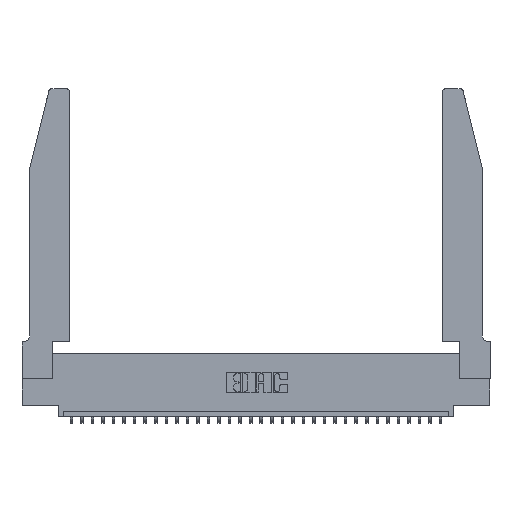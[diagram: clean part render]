
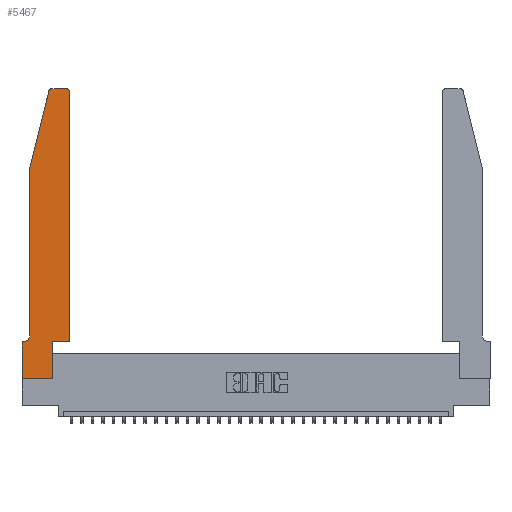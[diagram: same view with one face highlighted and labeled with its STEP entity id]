
A CAD part, top view. The second image highlights one B-rep face of the part: STEP entity #5467.
In plain terms, the highlighted planar face has unit normal (0, 0, 1).
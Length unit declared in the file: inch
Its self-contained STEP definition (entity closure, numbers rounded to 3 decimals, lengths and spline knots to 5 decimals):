
#91 = CARTESIAN_POINT ( 'NONE',  ( 0., 0., 0.37 ) ) ;
#189 = DIRECTION ( 'NONE',  ( 1., 0., 0. ) ) ;
#354 = VERTEX_POINT ( 'NONE', #4763 ) ;
#559 = AXIS2_PLACEMENT_3D ( 'NONE', #20808, #7820, #15425 ) ;
#624 = EDGE_CURVE ( 'NONE', #32583, #28221, #8043, .T. ) ;
#1134 = CARTESIAN_POINT ( 'NONE',  ( 0.2865, 0., 0.37 ) ) ;
#1502 = CARTESIAN_POINT ( 'NONE',  ( 0.284, 2.72, 0.37 ) ) ;
#1786 = AXIS2_PLACEMENT_3D ( 'NONE', #6317, #21742, #11799 ) ;
#2083 = CARTESIAN_POINT ( 'NONE',  ( 0.4505, 0.35, 0.37 ) ) ;
#2113 = EDGE_CURVE ( 'NONE', #14471, #32750, #32723, .T. ) ;
#2166 = DIRECTION ( 'NONE',  ( -1., 0., 0. ) ) ;
#2376 = CARTESIAN_POINT ( 'NONE',  ( 0.0755, 0.35, 0.37 ) ) ;
#2480 = CIRCLE ( 'NONE', #9374, 0.07 ) ;
#3508 = EDGE_CURVE ( 'NONE', #17828, #15352, #21882, .T. ) ;
#4002 = CIRCLE ( 'NONE', #26710, 0.03 ) ;
#4449 = CARTESIAN_POINT ( 'NONE',  ( 0.2865, 0.35, 0.37 ) ) ;
#4587 = VECTOR ( 'NONE', #30036, 39.37008 ) ;
#4680 = DIRECTION ( 'NONE',  ( 0., 1., 0. ) ) ;
#4698 = EDGE_CURVE ( 'NONE', #22124, #354, #21818, .T. ) ;
#4763 = CARTESIAN_POINT ( 'NONE',  ( 0.2865, 0.35, 0.37 ) ) ;
#5367 = CARTESIAN_POINT ( 'NONE',  ( 0.284, 2.75, 0.37 ) ) ;
#5467 = ADVANCED_FACE ( 'NONE', ( #28882 ), #31839, .T. ) ;
#5757 = ORIENTED_EDGE ( 'NONE', *, *, #4698, .T. ) ;
#6317 = CARTESIAN_POINT ( 'NONE',  ( 0., 0.35, 0.37 ) ) ;
#7056 = CARTESIAN_POINT ( 'NONE',  ( 0.4505, 0.35, 0.37 ) ) ;
#7820 = DIRECTION ( 'NONE',  ( 0., 0., 1. ) ) ;
#8043 = LINE ( 'NONE', #14419, #28275 ) ;
#8946 = VECTOR ( 'NONE', #189, 39.37008 ) ;
#9374 = AXIS2_PLACEMENT_3D ( 'NONE', #27541, #12500, #2166 ) ;
#9375 = LINE ( 'NONE', #2083, #4587 ) ;
#9387 = EDGE_CURVE ( 'NONE', #354, #25206, #22438, .T. ) ;
#9686 = CARTESIAN_POINT ( 'NONE',  ( 0., 0., 0.37 ) ) ;
#9742 = VECTOR ( 'NONE', #18309, 39.37008 ) ;
#9914 = DIRECTION ( 'NONE',  ( -1., 0., 0. ) ) ;
#9965 = DIRECTION ( 'NONE',  ( 0., 0., 1. ) ) ;
#10332 = ORIENTED_EDGE ( 'NONE', *, *, #15098, .T. ) ;
#10562 = DIRECTION ( 'NONE',  ( -0.239, -0.971, 0. ) ) ;
#10989 = ORIENTED_EDGE ( 'NONE', *, *, #12234, .T. ) ;
#11799 = DIRECTION ( 'NONE',  ( 1., 0., 0. ) ) ;
#12012 = DIRECTION ( 'NONE',  ( -1., 0., 0. ) ) ;
#12234 = EDGE_CURVE ( 'NONE', #12552, #17828, #25350, .T. ) ;
#12296 = DIRECTION ( 'NONE',  ( 1., 0., 0. ) ) ;
#12478 = VECTOR ( 'NONE', #10562, 39.37008 ) ;
#12500 = DIRECTION ( 'NONE',  ( 0., 0., -1. ) ) ;
#12552 = VERTEX_POINT ( 'NONE', #18207 ) ;
#13067 = EDGE_CURVE ( 'NONE', #15352, #14471, #4002, .T. ) ;
#14196 = DIRECTION ( 'NONE',  ( 0., -1., 0. ) ) ;
#14402 = ORIENTED_EDGE ( 'NONE', *, *, #3508, .T. ) ;
#14419 = CARTESIAN_POINT ( 'NONE',  ( 0., 0., 0.37 ) ) ;
#14471 = VERTEX_POINT ( 'NONE', #20940 ) ;
#15053 = ORIENTED_EDGE ( 'NONE', *, *, #9387, .T. ) ;
#15098 = EDGE_CURVE ( 'NONE', #25206, #12552, #9375, .T. ) ;
#15297 = ORIENTED_EDGE ( 'NONE', *, *, #17241, .T. ) ;
#15352 = VERTEX_POINT ( 'NONE', #5367 ) ;
#15425 = DIRECTION ( 'NONE',  ( 1., 0., 0. ) ) ;
#16119 = CARTESIAN_POINT ( 'NONE',  ( 0.4505, 0.35, 0.37 ) ) ;
#17241 = EDGE_CURVE ( 'NONE', #29196, #28815, #2480, .T. ) ;
#17347 = CARTESIAN_POINT ( 'NONE',  ( 0.0055, 0.35, 0.37 ) ) ;
#17789 = CARTESIAN_POINT ( 'NONE',  ( 0.4205, 2.75, 0.37 ) ) ;
#17828 = VERTEX_POINT ( 'NONE', #17789 ) ;
#18207 = CARTESIAN_POINT ( 'NONE',  ( 0.4505, 2.72, 0.37 ) ) ;
#18309 = DIRECTION ( 'NONE',  ( 0., -1., 0. ) ) ;
#18849 = CARTESIAN_POINT ( 'NONE',  ( 0., 0.35, 0.37 ) ) ;
#19034 = VECTOR ( 'NONE', #9914, 39.37008 ) ;
#19077 = VECTOR ( 'NONE', #4680, 39.37008 ) ;
#20066 = VECTOR ( 'NONE', #12296, 39.37008 ) ;
#20245 = DIRECTION ( 'NONE',  ( 1., 0., 0. ) ) ;
#20300 = EDGE_LOOP ( 'NONE', ( #14402, #24261, #25345, #27972, #15297, #26249, #27921, #20702, #5757, #15053, #10332, #10989 ) ) ;
#20441 = CARTESIAN_POINT ( 'NONE',  ( 0.0755, 2., 0.37 ) ) ;
#20702 = ORIENTED_EDGE ( 'NONE', *, *, #23317, .T. ) ;
#20808 = CARTESIAN_POINT ( 'NONE',  ( 0.4205, 2.72, 0.37 ) ) ;
#20824 = CARTESIAN_POINT ( 'NONE',  ( 0.0755, 2., 0.37 ) ) ;
#20940 = CARTESIAN_POINT ( 'NONE',  ( 0.25487, 2.72718, 0.37 ) ) ;
#21279 = EDGE_CURVE ( 'NONE', #28815, #32583, #29731, .T. ) ;
#21489 = CARTESIAN_POINT ( 'NONE',  ( 0.0755, 0.42, 0.37 ) ) ;
#21742 = DIRECTION ( 'NONE',  ( 0., 0., 1. ) ) ;
#21818 = LINE ( 'NONE', #4449, #19077 ) ;
#21882 = LINE ( 'NONE', #29264, #29422 ) ;
#22124 = VERTEX_POINT ( 'NONE', #1134 ) ;
#22438 = LINE ( 'NONE', #7056, #20066 ) ;
#23224 = LINE ( 'NONE', #20824, #9742 ) ;
#23306 = EDGE_CURVE ( 'NONE', #32750, #29196, #23224, .T. ) ;
#23317 = EDGE_CURVE ( 'NONE', #28221, #22124, #24844, .T. ) ;
#24261 = ORIENTED_EDGE ( 'NONE', *, *, #13067, .T. ) ;
#24844 = LINE ( 'NONE', #91, #8946 ) ;
#25206 = VERTEX_POINT ( 'NONE', #16119 ) ;
#25345 = ORIENTED_EDGE ( 'NONE', *, *, #2113, .T. ) ;
#25350 = CIRCLE ( 'NONE', #559, 0.03 ) ;
#26249 = ORIENTED_EDGE ( 'NONE', *, *, #21279, .T. ) ;
#26710 = AXIS2_PLACEMENT_3D ( 'NONE', #1502, #9965, #20245 ) ;
#27541 = CARTESIAN_POINT ( 'NONE',  ( 0.0055, 0.42, 0.37 ) ) ;
#27921 = ORIENTED_EDGE ( 'NONE', *, *, #624, .T. ) ;
#27972 = ORIENTED_EDGE ( 'NONE', *, *, #23306, .T. ) ;
#28221 = VERTEX_POINT ( 'NONE', #9686 ) ;
#28275 = VECTOR ( 'NONE', #14196, 39.37008 ) ;
#28815 = VERTEX_POINT ( 'NONE', #17347 ) ;
#28882 = FACE_OUTER_BOUND ( 'NONE', #20300, .T. ) ;
#29196 = VERTEX_POINT ( 'NONE', #21489 ) ;
#29264 = CARTESIAN_POINT ( 'NONE',  ( 0.2605, 2.75, 0.37 ) ) ;
#29422 = VECTOR ( 'NONE', #12012, 39.37008 ) ;
#29731 = LINE ( 'NONE', #2376, #19034 ) ;
#30036 = DIRECTION ( 'NONE',  ( 0., 1., 0. ) ) ;
#31701 = CARTESIAN_POINT ( 'NONE',  ( 0.0755, 2., 0.37 ) ) ;
#31839 = PLANE ( 'NONE',  #1786 ) ;
#32583 = VERTEX_POINT ( 'NONE', #18849 ) ;
#32723 = LINE ( 'NONE', #20441, #12478 ) ;
#32750 = VERTEX_POINT ( 'NONE', #31701 ) ;
